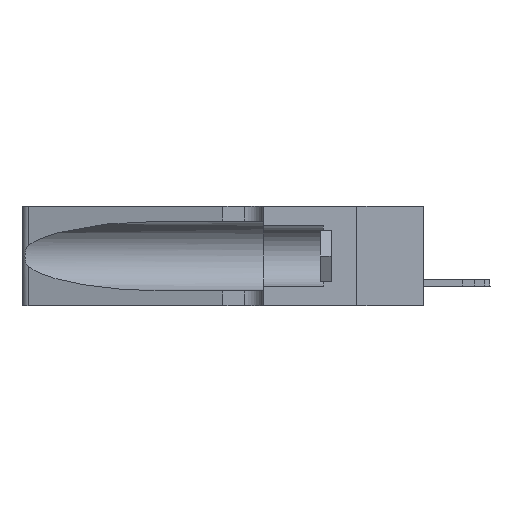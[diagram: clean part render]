
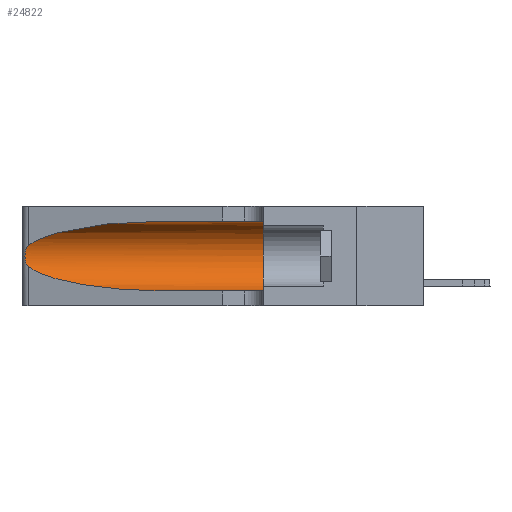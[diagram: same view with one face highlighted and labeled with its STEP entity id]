
A CAD part, left-side view. The second image highlights one B-rep face of the part: STEP entity #24822.
In plain terms, the highlighted cylindrical face has radius 3.308 mm (diameter 6.617 mm), a partial arc.
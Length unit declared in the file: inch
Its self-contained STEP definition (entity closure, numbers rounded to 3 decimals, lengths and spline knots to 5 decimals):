
#1028 = CARTESIAN_POINT ( 'NONE',  ( 0.2373, 1.15595, 0.08982 ) ) ;
#1387 = CARTESIAN_POINT ( 'NONE',  ( 0.25555, 1.22994, 0.2215 ) ) ;
#1681 = CARTESIAN_POINT ( 'NONE',  ( 0.18966, 0.96281, 0.05475 ) ) ;
#2113 = CARTESIAN_POINT ( 'NONE',  ( 0.25639, 1.23186, 0.15144 ) ) ;
#2200 = VERTEX_POINT ( 'NONE', #10386 ) ;
#3031 = ORIENTED_EDGE ( 'NONE', *, *, #24875, .T. ) ;
#3949 = DIRECTION ( 'NONE',  ( 0., -1., 0. ) ) ;
#4023 = CARTESIAN_POINT ( 'NONE',  ( 0.26075, 1.23896, 0.19203 ) ) ;
#4593 = CARTESIAN_POINT ( 'NONE',  ( 0.1305, 0.72297, 0.31525 ) ) ;
#5632 = CARTESIAN_POINT ( 'NONE',  ( 0.1305, 1.61858, 0.31525 ) ) ;
#5642 = VECTOR ( 'NONE', #21511, 39.37008 ) ;
#6346 = CARTESIAN_POINT ( 'NONE',  ( 0.25487, 1.22718, 0.22369 ) ) ;
#6371 = B_SPLINE_CURVE_WITH_KNOTS ( 'NONE', 3,
 ( #6346, #1387, #30335, #30221, #27774, #17160, #4023, #27530, #32437, #17593, #12321, #2113, #18895, #26937 ),
 .UNSPECIFIED., .F., .F.,
 ( 4, 2, 2, 2, 2, 2, 4 ),
 ( 0., 0.00027, 0.00053, 0.00107, 0.0016, 0.00187, 0.00214 ),
 .UNSPECIFIED. ) ;
#6934 = ORIENTED_EDGE ( 'NONE', *, *, #23165, .F. ) ;
#7347 = LINE ( 'NONE', #5632, #5642 ) ;
#7387 = VERTEX_POINT ( 'NONE', #4593 ) ;
#7578 = VECTOR ( 'NONE', #20089, 39.37008 ) ;
#8919 = CARTESIAN_POINT ( 'NONE',  ( 0.1305, 0.72297, 0.31525 ) ) ;
#9144 = CARTESIAN_POINT ( 'NONE',  ( 0.1305, 1.61858, 0.05475 ) ) ;
#9946 = AXIS2_PLACEMENT_3D ( 'NONE', #20451, #33779, #20683 ) ;
#10386 = CARTESIAN_POINT ( 'NONE',  ( 0.1305, 0.35, 0.31525 ) ) ;
#11171 = EDGE_CURVE ( 'NONE', #12221, #20264, #6371, .T. ) ;
#11179 = EDGE_CURVE ( 'NONE', #20264, #24990, #12991, .T. ) ;
#11213 = ORIENTED_EDGE ( 'NONE', *, *, #11179, .T. ) ;
#12221 = VERTEX_POINT ( 'NONE', #22700 ) ;
#12321 = CARTESIAN_POINT ( 'NONE',  ( 0.25789, 1.23486, 0.15765 ) ) ;
#12967 = LINE ( 'NONE', #9144, #7578 ) ;
#12991 =( BOUNDED_CURVE ( )  B_SPLINE_CURVE ( 3, ( #19127, #1028, #1681, #22391 ),
 .UNSPECIFIED., .F., .F. ) 
 B_SPLINE_CURVE_WITH_KNOTS ( ( 4, 4 ),
 ( 3.44316, 4.71239 ),
 .UNSPECIFIED. ) 
 CURVE ( )  GEOMETRIC_REPRESENTATION_ITEM ( )  RATIONAL_B_SPLINE_CURVE ( ( 1., 0.87, 0.87, 1. ) ) 
 REPRESENTATION_ITEM ( '' )  );
#14405 = CARTESIAN_POINT ( 'NONE',  ( 0.1305, 1.61858, 0.185 ) ) ;
#17160 = CARTESIAN_POINT ( 'NONE',  ( 0.26018, 1.23835, 0.19895 ) ) ;
#17593 = CARTESIAN_POINT ( 'NONE',  ( 0.25856, 1.23593, 0.16098 ) ) ;
#18895 = CARTESIAN_POINT ( 'NONE',  ( 0.25555, 1.22993, 0.14849 ) ) ;
#19127 = CARTESIAN_POINT ( 'NONE',  ( 0.25487, 1.22718, 0.14631 ) ) ;
#19347 = ORIENTED_EDGE ( 'NONE', *, *, #22018, .F. ) ;
#20089 = DIRECTION ( 'NONE',  ( 0., -1., 0. ) ) ;
#20264 = VERTEX_POINT ( 'NONE', #20839 ) ;
#20451 = CARTESIAN_POINT ( 'NONE',  ( 0.1305, 0.35, 0.185 ) ) ;
#20683 = DIRECTION ( 'NONE',  ( 0., 0., 1. ) ) ;
#20839 = CARTESIAN_POINT ( 'NONE',  ( 0.25487, 1.22718, 0.14631 ) ) ;
#21250 =( BOUNDED_CURVE ( )  B_SPLINE_CURVE ( 3, ( #8919, #27479, #32834, #32496 ),
 .UNSPECIFIED., .F., .F. ) 
 B_SPLINE_CURVE_WITH_KNOTS ( ( 4, 4 ),
 ( 1.5708, 2.84003 ),
 .UNSPECIFIED. ) 
 CURVE ( )  GEOMETRIC_REPRESENTATION_ITEM ( )  RATIONAL_B_SPLINE_CURVE ( ( 1., 0.87, 0.87, 1. ) ) 
 REPRESENTATION_ITEM ( '' )  );
#21511 = DIRECTION ( 'NONE',  ( 0., -1., 0. ) ) ;
#22018 = EDGE_CURVE ( 'NONE', #7387, #2200, #7347, .T. ) ;
#22391 = CARTESIAN_POINT ( 'NONE',  ( 0.1305, 0.72297, 0.05475 ) ) ;
#22608 = ORIENTED_EDGE ( 'NONE', *, *, #27677, .T. ) ;
#22700 = CARTESIAN_POINT ( 'NONE',  ( 0.25487, 1.22718, 0.22369 ) ) ;
#23165 = EDGE_CURVE ( 'NONE', #2200, #33671, #26662, .T. ) ;
#24822 = ADVANCED_FACE ( 'NONE', ( #30382 ), #29979, .F. ) ;
#24875 = EDGE_CURVE ( 'NONE', #24990, #33671, #12967, .T. ) ;
#24990 = VERTEX_POINT ( 'NONE', #25871 ) ;
#25287 = DIRECTION ( 'NONE',  ( 0., 0., -1. ) ) ;
#25871 = CARTESIAN_POINT ( 'NONE',  ( 0.1305, 0.72297, 0.05475 ) ) ;
#26662 = CIRCLE ( 'NONE', #9946, 0.13025 ) ;
#26937 = CARTESIAN_POINT ( 'NONE',  ( 0.25487, 1.22718, 0.14631 ) ) ;
#27479 = CARTESIAN_POINT ( 'NONE',  ( 0.18966, 0.96281, 0.31525 ) ) ;
#27530 = CARTESIAN_POINT ( 'NONE',  ( 0.26075, 1.23896, 0.178 ) ) ;
#27677 = EDGE_CURVE ( 'NONE', #7387, #12221, #21250, .T. ) ;
#27774 = CARTESIAN_POINT ( 'NONE',  ( 0.25854, 1.2359, 0.20912 ) ) ;
#29513 = EDGE_LOOP ( 'NONE', ( #22608, #30815, #11213, #3031, #6934, #19347 ) ) ;
#29979 = CYLINDRICAL_SURFACE ( 'NONE', #33327, 0.13025 ) ;
#30221 = CARTESIAN_POINT ( 'NONE',  ( 0.25787, 1.23484, 0.2124 ) ) ;
#30335 = CARTESIAN_POINT ( 'NONE',  ( 0.25639, 1.23184, 0.21858 ) ) ;
#30382 = FACE_OUTER_BOUND ( 'NONE', #29513, .T. ) ;
#30815 = ORIENTED_EDGE ( 'NONE', *, *, #11171, .T. ) ;
#32437 = CARTESIAN_POINT ( 'NONE',  ( 0.26017, 1.23833, 0.17102 ) ) ;
#32496 = CARTESIAN_POINT ( 'NONE',  ( 0.25487, 1.22718, 0.22369 ) ) ;
#32834 = CARTESIAN_POINT ( 'NONE',  ( 0.2373, 1.15595, 0.28018 ) ) ;
#33327 = AXIS2_PLACEMENT_3D ( 'NONE', #14405, #3949, #25287 ) ;
#33671 = VERTEX_POINT ( 'NONE', #34128 ) ;
#33779 = DIRECTION ( 'NONE',  ( 0., 1., 0. ) ) ;
#34128 = CARTESIAN_POINT ( 'NONE',  ( 0.1305, 0.35, 0.05475 ) ) ;
